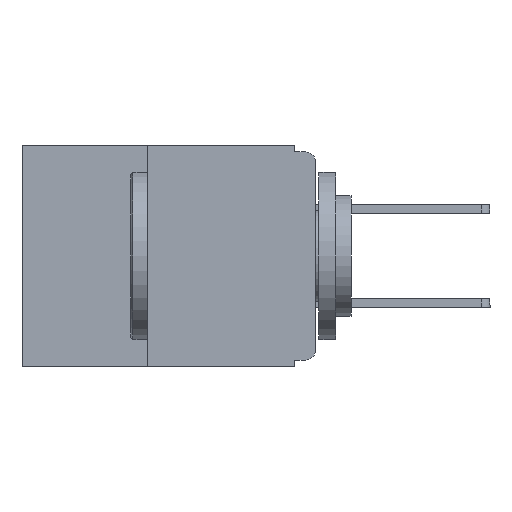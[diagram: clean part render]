
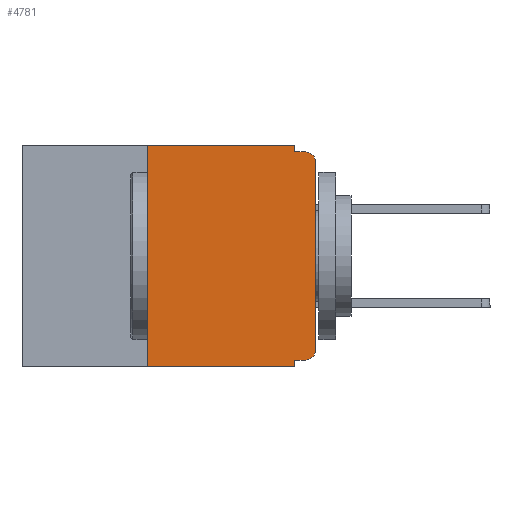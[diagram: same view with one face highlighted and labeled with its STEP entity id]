
A CAD part, left-side view. The second image highlights one B-rep face of the part: STEP entity #4781.
In plain terms, the highlighted planar face has unit normal (-1, 0, 0).
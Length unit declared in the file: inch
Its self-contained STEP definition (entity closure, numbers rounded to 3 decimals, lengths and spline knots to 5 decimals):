
#69 = EDGE_CURVE ( 'NONE', #4143, #28370, #29281, .T. ) ;
#160 = CIRCLE ( 'NONE', #11303, 0.015 ) ;
#337 = ORIENTED_EDGE ( 'NONE', *, *, #9726, .F. ) ;
#499 = ORIENTED_EDGE ( 'NONE', *, *, #69, .T. ) ;
#621 = CARTESIAN_POINT ( 'NONE',  ( 0., 0.015, -0.32 ) ) ;
#693 = EDGE_CURVE ( 'NONE', #20590, #4143, #24777, .T. ) ;
#1138 = DIRECTION ( 'NONE',  ( 0., 0., -1. ) ) ;
#2495 = DIRECTION ( 'NONE',  ( 0., 0., -1. ) ) ;
#2976 = DIRECTION ( 'NONE',  ( 0., 1., 0. ) ) ;
#3965 = EDGE_CURVE ( 'NONE', #28370, #20477, #160, .T. ) ;
#4143 = VERTEX_POINT ( 'NONE', #16536 ) ;
#4340 = VECTOR ( 'NONE', #28120, 39.37008 ) ;
#4659 = EDGE_CURVE ( 'NONE', #13807, #4725, #31245, .T. ) ;
#4725 = VERTEX_POINT ( 'NONE', #23383 ) ;
#4781 = ADVANCED_FACE ( 'NONE', ( #14721 ), #22095, .F. ) ;
#5106 = LINE ( 'NONE', #13703, #4340 ) ;
#5144 = DIRECTION ( 'NONE',  ( 0., 0., 1. ) ) ;
#5649 = VECTOR ( 'NONE', #2495, 39.37008 ) ;
#5755 = VECTOR ( 'NONE', #5144, 39.37008 ) ;
#6273 = ORIENTED_EDGE ( 'NONE', *, *, #14673, .F. ) ;
#7477 = CARTESIAN_POINT ( 'NONE',  ( 0., 0.015, -0.01 ) ) ;
#7570 = LINE ( 'NONE', #17631, #20551 ) ;
#7815 = AXIS2_PLACEMENT_3D ( 'NONE', #21920, #21614, #21586 ) ;
#9347 = ORIENTED_EDGE ( 'NONE', *, *, #20356, .F. ) ;
#9378 = ORIENTED_EDGE ( 'NONE', *, *, #11365, .T. ) ;
#9442 = CARTESIAN_POINT ( 'NONE',  ( 0., 0., -0.01 ) ) ;
#9726 = EDGE_CURVE ( 'NONE', #25273, #16274, #12212, .T. ) ;
#9833 = VECTOR ( 'NONE', #10986, 39.37008 ) ;
#9878 = CARTESIAN_POINT ( 'NONE',  ( 0., 0.25, -0.33 ) ) ;
#10393 = DIRECTION ( 'NONE',  ( 0., 0., 1. ) ) ;
#10550 = EDGE_CURVE ( 'NONE', #20590, #25273, #7570, .T. ) ;
#10588 = LINE ( 'NONE', #25538, #9833 ) ;
#10964 = CARTESIAN_POINT ( 'NONE',  ( 0., 0., 0. ) ) ;
#10986 = DIRECTION ( 'NONE',  ( 0., -1., 0. ) ) ;
#11303 = AXIS2_PLACEMENT_3D ( 'NONE', #28349, #28121, #27886 ) ;
#11365 = EDGE_CURVE ( 'NONE', #22331, #16274, #10588, .T. ) ;
#12032 = VECTOR ( 'NONE', #24634, 39.37008 ) ;
#12212 = LINE ( 'NONE', #12308, #5649 ) ;
#12308 = CARTESIAN_POINT ( 'NONE',  ( 0., 0.031, -0.33 ) ) ;
#12317 = LINE ( 'NONE', #26975, #5755 ) ;
#12686 = AXIS2_PLACEMENT_3D ( 'NONE', #23901, #17829, #1138 ) ;
#12774 = CARTESIAN_POINT ( 'NONE',  ( 0., 0.031, -0.32 ) ) ;
#13032 = ORIENTED_EDGE ( 'NONE', *, *, #693, .T. ) ;
#13063 = ORIENTED_EDGE ( 'NONE', *, *, #10550, .F. ) ;
#13703 = CARTESIAN_POINT ( 'NONE',  ( 0., 0.031, 0. ) ) ;
#13807 = VERTEX_POINT ( 'NONE', #16659 ) ;
#14673 = EDGE_CURVE ( 'NONE', #22331, #13807, #12317, .T. ) ;
#14721 = FACE_OUTER_BOUND ( 'NONE', #24985, .T. ) ;
#15671 = CARTESIAN_POINT ( 'NONE',  ( 0., 0.031, -0.01 ) ) ;
#16252 = EDGE_CURVE ( 'NONE', #4725, #24419, #5106, .T. ) ;
#16274 = VERTEX_POINT ( 'NONE', #23382 ) ;
#16536 = CARTESIAN_POINT ( 'NONE',  ( 0., 0., -0.305 ) ) ;
#16659 = CARTESIAN_POINT ( 'NONE',  ( 0., 0.25, 0. ) ) ;
#17333 = ORIENTED_EDGE ( 'NONE', *, *, #16252, .F. ) ;
#17631 = CARTESIAN_POINT ( 'NONE',  ( 0., 0., -0.32 ) ) ;
#17829 = DIRECTION ( 'NONE',  ( -1., 0., 0. ) ) ;
#19769 = VECTOR ( 'NONE', #28797, 39.37008 ) ;
#20356 = EDGE_CURVE ( 'NONE', #24419, #20477, #26921, .T. ) ;
#20404 = ORIENTED_EDGE ( 'NONE', *, *, #4659, .F. ) ;
#20477 = VERTEX_POINT ( 'NONE', #7477 ) ;
#20551 = VECTOR ( 'NONE', #2976, 39.37008 ) ;
#20590 = VERTEX_POINT ( 'NONE', #621 ) ;
#21508 = ORIENTED_EDGE ( 'NONE', *, *, #3965, .T. ) ;
#21586 = DIRECTION ( 'NONE',  ( 0., 0., -1. ) ) ;
#21614 = DIRECTION ( 'NONE',  ( 1., 0., 0. ) ) ;
#21920 = CARTESIAN_POINT ( 'NONE',  ( 0., 0.437, 0. ) ) ;
#22095 = PLANE ( 'NONE',  #7815 ) ;
#22331 = VERTEX_POINT ( 'NONE', #9878 ) ;
#22916 = VECTOR ( 'NONE', #10393, 39.37008 ) ;
#23382 = CARTESIAN_POINT ( 'NONE',  ( 0., 0.031, -0.33 ) ) ;
#23383 = CARTESIAN_POINT ( 'NONE',  ( 0., 0.031, 0. ) ) ;
#23901 = CARTESIAN_POINT ( 'NONE',  ( 0., 0.015, -0.305 ) ) ;
#24419 = VERTEX_POINT ( 'NONE', #15671 ) ;
#24629 = CARTESIAN_POINT ( 'NONE',  ( 0., 0.437, 0. ) ) ;
#24634 = DIRECTION ( 'NONE',  ( 0., -1., 0. ) ) ;
#24777 = CIRCLE ( 'NONE', #12686, 0.015 ) ;
#24985 = EDGE_LOOP ( 'NONE', ( #499, #21508, #9347, #17333, #20404, #6273, #9378, #337, #13063, #13032 ) ) ;
#25273 = VERTEX_POINT ( 'NONE', #12774 ) ;
#25538 = CARTESIAN_POINT ( 'NONE',  ( 0., 0.437, -0.33 ) ) ;
#26921 = LINE ( 'NONE', #9442, #19769 ) ;
#26975 = CARTESIAN_POINT ( 'NONE',  ( 0., 0.25, -0.33 ) ) ;
#27886 = DIRECTION ( 'NONE',  ( 0., 0., -1. ) ) ;
#28120 = DIRECTION ( 'NONE',  ( 0., 0., -1. ) ) ;
#28121 = DIRECTION ( 'NONE',  ( -1., 0., 0. ) ) ;
#28349 = CARTESIAN_POINT ( 'NONE',  ( 0., 0.015, -0.025 ) ) ;
#28370 = VERTEX_POINT ( 'NONE', #31236 ) ;
#28797 = DIRECTION ( 'NONE',  ( 0., -1., 0. ) ) ;
#29281 = LINE ( 'NONE', #10964, #22916 ) ;
#31236 = CARTESIAN_POINT ( 'NONE',  ( 0., 0., -0.025 ) ) ;
#31245 = LINE ( 'NONE', #24629, #12032 ) ;
